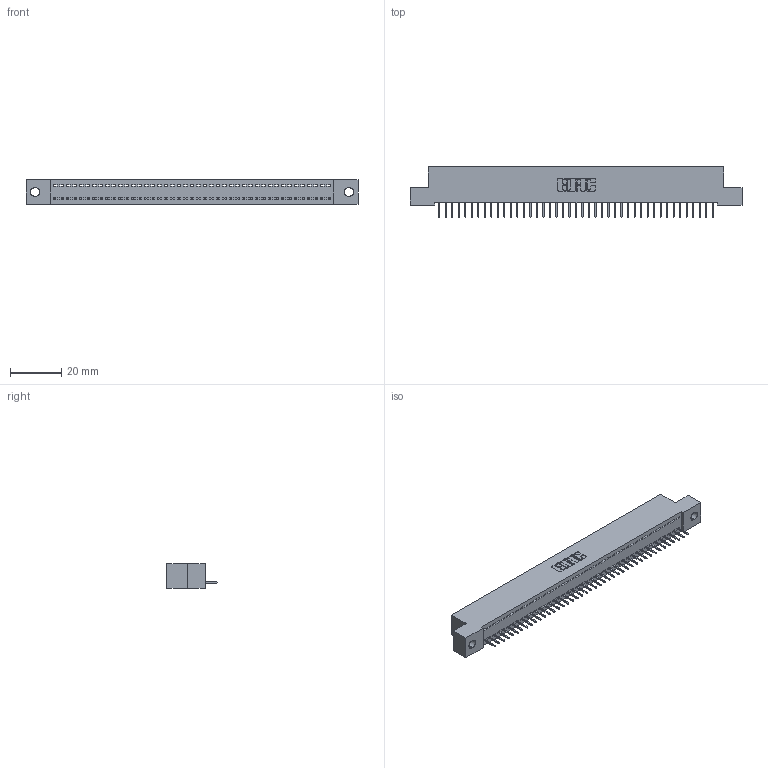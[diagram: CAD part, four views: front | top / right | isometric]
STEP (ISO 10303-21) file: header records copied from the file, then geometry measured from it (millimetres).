
FILE_DESCRIPTION (( 'STEP AP203' ), '1' );
FILE_NAME ('392-043-524-102.STEP', '2019-10-07T21:41:42', ( '' ), ( '' ), 'SwSTEP 2.0', 'SolidWorks 2016', '' );
FILE_SCHEMA (( 'CONFIG_CONTROL_DESIGN' ));
Length unit declared in the file: inch
Products named in the file (3): 342 Part_.128 Slot; 345-292-001_345-293-124; 392-043-524-102
Assembly tree (44 placements, depth 2):
  392-043-524-102
    342 Part_.128 Slot
    345-292-001_345-293-124  x43
Bounding box: 129.54 x 19.69 x 9.4 mm (x, y, z)
Volume: 11139.7 mm3; surface area: 15608.9 mm2
Topology: 44 solids, 44 shells, 2780 faces, 8051 edges, 5194 vertices
Faces by surface type: plane 2134, cylinder 646
Entity records: 26235 total; most frequent: CARTESIAN_POINT 4531, ORIENTED_EDGE 4510, DIRECTION 3821, EDGE_CURVE 2255, VECTOR 2131, LINE 2131, VERTEX_POINT 1498, AXIS2_PLACEMENT_3D 845
